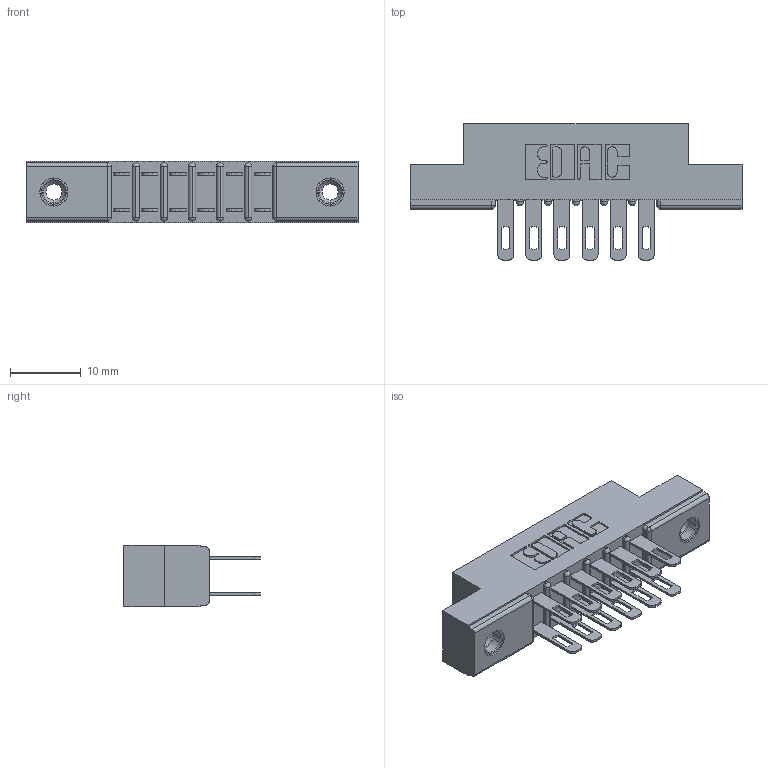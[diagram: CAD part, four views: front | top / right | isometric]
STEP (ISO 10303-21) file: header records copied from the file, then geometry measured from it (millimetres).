
FILE_DESCRIPTION (( 'STEP AP203' ), '1' );
FILE_NAME ('357-012-400-208.STEP', '2020-10-02T15:53:57', ( '' ), ( '' ), 'SwSTEP 2.0', 'SolidWorks 2020', '' );
FILE_SCHEMA (( 'CONFIG_CONTROL_DESIGN' ));
Length unit declared in the file: inch
Products named in the file (4): 307-290-001_500; 307 Part_.156 Dia Mounting Holes; 357-012-400-208; 345-250-001_345-250-003-102
Assembly tree (15 placements, depth 2):
  357-012-400-208
    307 Part_.156 Dia Mounting Holes
    307-290-001_500  x12
    345-250-001_345-250-003-102  x2
Bounding box: 46.79 x 19.18 x 8.71 mm (x, y, z)
Volume: 3090 mm3; surface area: 4835.7 mm2
Topology: 15 solids, 15 shells, 737 faces, 2019 edges, 1302 vertices
Faces by surface type: plane 462, cylinder 245, sphere 14, cone 12, torus 4
Entity records: 10933 total; most frequent: CARTESIAN_POINT 1781, DIRECTION 1771, ORIENTED_EDGE 1754, EDGE_CURVE 877, LINE 655, VECTOR 655, VERTEX_POINT 568, AXIS2_PLACEMENT_3D 558
